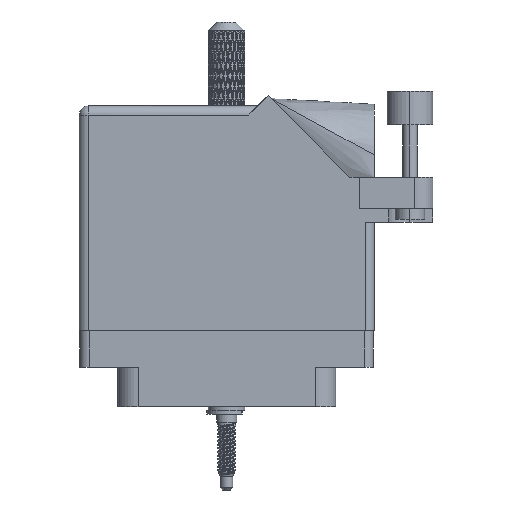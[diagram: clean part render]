
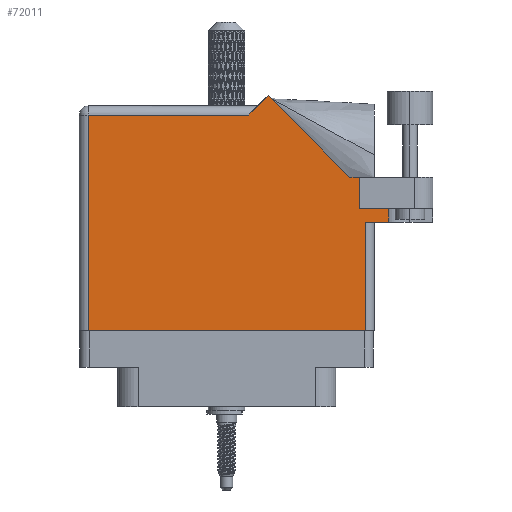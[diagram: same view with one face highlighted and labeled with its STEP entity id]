
A CAD part, front view. The second image highlights one B-rep face of the part: STEP entity #72011.
In plain terms, the highlighted face is planar.
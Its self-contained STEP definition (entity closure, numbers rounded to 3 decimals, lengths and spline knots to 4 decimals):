
#473 = DIRECTION ( 'NONE',  ( 0., -1., 0. ) ) ;
#2520 = VERTEX_POINT ( 'NONE', #37414 ) ;
#5535 = CARTESIAN_POINT ( 'NONE',  ( 0.905, 0.731, 0.455 ) ) ;
#7579 = VECTOR ( 'NONE', #94981, 39.3701 ) ;
#8514 = CARTESIAN_POINT ( 'NONE',  ( -1.005, -0.1, 0.455 ) ) ;
#10243 = CARTESIAN_POINT ( 'NONE',  ( 0.943, 0.637, 0.455 ) ) ;
#10246 = CARTESIAN_POINT ( 'NONE',  ( -0.943, 1.368, 0.455 ) ) ;
#11498 = CARTESIAN_POINT ( 'NONE',  ( 0.15, 1.368, 0.455 ) ) ;
#13880 = ORIENTED_EDGE ( 'NONE', *, *, #61094, .T. ) ;
#15241 = LINE ( 'NONE', #32431, #64062 ) ;
#16222 = LINE ( 'NONE', #5535, #45795 ) ;
#18113 = AXIS2_PLACEMENT_3D ( 'NONE', #31958, #23344, #22297 ) ;
#18587 = EDGE_CURVE ( 'NONE', #85572, #86522, #29453, .T. ) ;
#20725 = ORIENTED_EDGE ( 'NONE', *, *, #92552, .T. ) ;
#21387 = CARTESIAN_POINT ( 'NONE',  ( 1.1065, 0.731, 0.455 ) ) ;
#21394 = DIRECTION ( 'NONE',  ( 1., 0., 0. ) ) ;
#22297 = DIRECTION ( 'NONE',  ( -1., 0., 0. ) ) ;
#23336 = LINE ( 'NONE', #48500, #54043 ) ;
#23344 = DIRECTION ( 'NONE',  ( 0., 0., -1. ) ) ;
#28226 = EDGE_CURVE ( 'NONE', #40181, #54006, #92782, .T. ) ;
#28303 = CARTESIAN_POINT ( 'NONE',  ( 0.8394, 0.944, 0.455 ) ) ;
#29453 = LINE ( 'NONE', #30568, #7579 ) ;
#30568 = CARTESIAN_POINT ( 'NONE',  ( 0.905, 0.731, 0.455 ) ) ;
#31641 = CARTESIAN_POINT ( 'NONE',  ( 0.905, 0.944, 0.455 ) ) ;
#31958 = CARTESIAN_POINT ( 'NONE',  ( -1.005, 1.43, 0.455 ) ) ;
#32431 = CARTESIAN_POINT ( 'NONE',  ( 1.1065, 1.0618, 0.455 ) ) ;
#35823 = EDGE_CURVE ( 'NONE', #45294, #2520, #57313, .T. ) ;
#36935 = VERTEX_POINT ( 'NONE', #57761 ) ;
#37414 = CARTESIAN_POINT ( 'NONE',  ( -0.943, -0.1, 0.455 ) ) ;
#37608 = EDGE_CURVE ( 'NONE', #85572, #40181, #16222, .T. ) ;
#40181 = VERTEX_POINT ( 'NONE', #31641 ) ;
#40246 = VECTOR ( 'NONE', #47084, 39.3701 ) ;
#40856 = CARTESIAN_POINT ( 'NONE',  ( 0.8394, 0.944, 0.455 ) ) ;
#41082 = CARTESIAN_POINT ( 'NONE',  ( -1.005, 1.368, 0.455 ) ) ;
#41860 = VERTEX_POINT ( 'NONE', #10243 ) ;
#45294 = VERTEX_POINT ( 'NONE', #10246 ) ;
#45660 = DIRECTION ( 'NONE',  ( -0.707, -0.707, 0. ) ) ;
#45795 = VECTOR ( 'NONE', #60002, 39.3701 ) ;
#47084 = DIRECTION ( 'NONE',  ( -1., 0., 0. ) ) ;
#48020 = VERTEX_POINT ( 'NONE', #50016 ) ;
#48500 = CARTESIAN_POINT ( 'NONE',  ( 0.943, 0.637, 0.455 ) ) ;
#49286 = DIRECTION ( 'NONE',  ( -1., 0., 0. ) ) ;
#49573 = CARTESIAN_POINT ( 'NONE',  ( -0.943, -0.1, 0.455 ) ) ;
#50016 = CARTESIAN_POINT ( 'NONE',  ( 0.943, -0.1, 0.455 ) ) ;
#50516 = EDGE_CURVE ( 'NONE', #54006, #57876, #92223, .T. ) ;
#51763 = CARTESIAN_POINT ( 'NONE',  ( 0.905, 0.731, 0.455 ) ) ;
#52481 = CARTESIAN_POINT ( 'NONE',  ( 0.212, 1.43, 0.455 ) ) ;
#53202 = LINE ( 'NONE', #8514, #72453 ) ;
#54006 = VERTEX_POINT ( 'NONE', #28303 ) ;
#54043 = VECTOR ( 'NONE', #57168, 39.3701 ) ;
#55120 = ORIENTED_EDGE ( 'NONE', *, *, #100404, .F. ) ;
#55734 = DIRECTION ( 'NONE',  ( 0., -1., 0. ) ) ;
#57043 = DIRECTION ( 'NONE',  ( -0.707, 0.707, 0. ) ) ;
#57158 = VECTOR ( 'NONE', #49286, 39.3701 ) ;
#57168 = DIRECTION ( 'NONE',  ( 0., 1., 0. ) ) ;
#57313 = LINE ( 'NONE', #49573, #91877 ) ;
#57655 = VECTOR ( 'NONE', #57043, 39.3701 ) ;
#57761 = CARTESIAN_POINT ( 'NONE',  ( 1.1065, 0.637, 0.455 ) ) ;
#57876 = VERTEX_POINT ( 'NONE', #102208 ) ;
#59003 = ORIENTED_EDGE ( 'NONE', *, *, #18587, .F. ) ;
#60002 = DIRECTION ( 'NONE',  ( 0., 1., 0. ) ) ;
#61094 = EDGE_CURVE ( 'NONE', #48020, #41860, #23336, .T. ) ;
#63286 = VERTEX_POINT ( 'NONE', #11498 ) ;
#63899 = ORIENTED_EDGE ( 'NONE', *, *, #35823, .T. ) ;
#64062 = VECTOR ( 'NONE', #55734, 39.3701 ) ;
#66313 = ORIENTED_EDGE ( 'NONE', *, *, #50516, .T. ) ;
#70530 = CARTESIAN_POINT ( 'NONE',  ( 1.005, 0.637, 0.455 ) ) ;
#72011 = ADVANCED_FACE ( 'NONE', ( #101470 ), #96363, .F. ) ;
#72453 = VECTOR ( 'NONE', #82686, 39.3701 ) ;
#75811 = ORIENTED_EDGE ( 'NONE', *, *, #90060, .T. ) ;
#76500 = VECTOR ( 'NONE', #21394, 39.3701 ) ;
#76952 = VECTOR ( 'NONE', #45660, 39.3701 ) ;
#78138 = LINE ( 'NONE', #52481, #76952 ) ;
#80042 = CARTESIAN_POINT ( 'NONE',  ( 1.405, 0.944, 0.455 ) ) ;
#82686 = DIRECTION ( 'NONE',  ( 1., 0., 0. ) ) ;
#83531 = EDGE_CURVE ( 'NONE', #63286, #45294, #103187, .T. ) ;
#85572 = VERTEX_POINT ( 'NONE', #51763 ) ;
#86522 = VERTEX_POINT ( 'NONE', #21387 ) ;
#89271 = LINE ( 'NONE', #70530, #76500 ) ;
#90060 = EDGE_CURVE ( 'NONE', #57876, #63286, #78138, .T. ) ;
#91877 = VECTOR ( 'NONE', #473, 39.3701 ) ;
#92223 = LINE ( 'NONE', #40856, #57655 ) ;
#92552 = EDGE_CURVE ( 'NONE', #41860, #36935, #89271, .T. ) ;
#92782 = LINE ( 'NONE', #80042, #40246 ) ;
#93707 = EDGE_CURVE ( 'NONE', #2520, #48020, #53202, .T. ) ;
#94038 = ORIENTED_EDGE ( 'NONE', *, *, #28226, .T. ) ;
#94981 = DIRECTION ( 'NONE',  ( 1., 0., 0. ) ) ;
#95009 = ORIENTED_EDGE ( 'NONE', *, *, #93707, .T. ) ;
#96363 = PLANE ( 'NONE',  #18113 ) ;
#98281 = ORIENTED_EDGE ( 'NONE', *, *, #83531, .T. ) ;
#99172 = EDGE_LOOP ( 'NONE', ( #95009, #13880, #20725, #55120, #59003, #106260, #94038, #66313, #75811, #98281, #63899 ) ) ;
#100404 = EDGE_CURVE ( 'NONE', #86522, #36935, #15241, .T. ) ;
#101470 = FACE_OUTER_BOUND ( 'NONE', #99172, .T. ) ;
#102208 = CARTESIAN_POINT ( 'NONE',  ( 0.2827, 1.5007, 0.455 ) ) ;
#103187 = LINE ( 'NONE', #41082, #57158 ) ;
#106260 = ORIENTED_EDGE ( 'NONE', *, *, #37608, .T. ) ;
